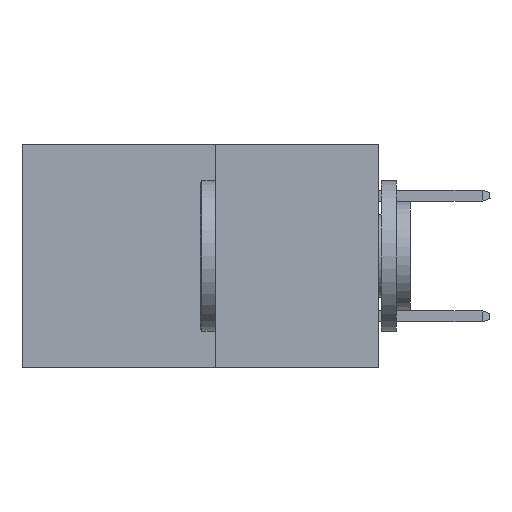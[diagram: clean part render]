
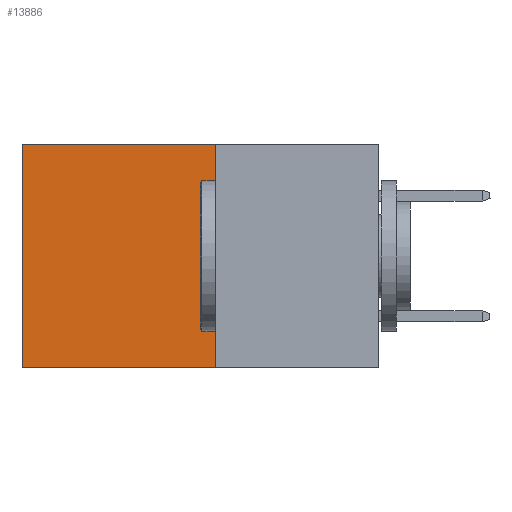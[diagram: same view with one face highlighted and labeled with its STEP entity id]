
A CAD part, left-side view. The second image highlights one B-rep face of the part: STEP entity #13886.
In plain terms, the highlighted planar face has unit normal (-1, 0, 0).
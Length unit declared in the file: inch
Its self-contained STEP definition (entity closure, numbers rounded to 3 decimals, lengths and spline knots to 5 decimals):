
#394 = AXIS2_PLACEMENT_3D ( 'NONE', #7461, #22733, #7569 ) ;
#2318 = CARTESIAN_POINT ( 'NONE',  ( 0.277, 0.59, -0.37 ) ) ;
#2329 = LINE ( 'NONE', #16534, #15059 ) ;
#3962 = ORIENTED_EDGE ( 'NONE', *, *, #25632, .T. ) ;
#4520 = ORIENTED_EDGE ( 'NONE', *, *, #11600, .T. ) ;
#5054 = PLANE ( 'NONE',  #394 ) ;
#7461 = CARTESIAN_POINT ( 'NONE',  ( 0.277, 0.27, -0.37 ) ) ;
#7485 = EDGE_CURVE ( 'NONE', #15143, #20458, #16448, .T. ) ;
#7569 = DIRECTION ( 'NONE',  ( 0., 0., -1. ) ) ;
#7715 = CARTESIAN_POINT ( 'NONE',  ( 0.277, 0.27, -0.37 ) ) ;
#9177 = DIRECTION ( 'NONE',  ( 0., 1., 0. ) ) ;
#9205 = LINE ( 'NONE', #21121, #28541 ) ;
#11600 = EDGE_CURVE ( 'NONE', #23104, #20458, #2329, .T. ) ;
#11608 = DIRECTION ( 'NONE',  ( 0., 0., -1. ) ) ;
#12657 = LINE ( 'NONE', #24418, #13428 ) ;
#12912 = VERTEX_POINT ( 'NONE', #16343 ) ;
#12972 = EDGE_LOOP ( 'NONE', ( #4520, #27186, #19836, #3962 ) ) ;
#13075 = DIRECTION ( 'NONE',  ( 0., 1., 0. ) ) ;
#13182 = CARTESIAN_POINT ( 'NONE',  ( 0.277, 0.27, -0.37 ) ) ;
#13428 = VECTOR ( 'NONE', #9177, 39.37008 ) ;
#13886 = ADVANCED_FACE ( 'NONE', ( #32751 ), #5054, .F. ) ;
#15059 = VECTOR ( 'NONE', #11608, 39.37008 ) ;
#15143 = VERTEX_POINT ( 'NONE', #7715 ) ;
#16343 = CARTESIAN_POINT ( 'NONE',  ( 0.277, 0.27, 0. ) ) ;
#16398 = CARTESIAN_POINT ( 'NONE',  ( 0.277, 0.59, 0. ) ) ;
#16448 = LINE ( 'NONE', #13182, #29089 ) ;
#16534 = CARTESIAN_POINT ( 'NONE',  ( 0.277, 0.59, -0.37 ) ) ;
#19836 = ORIENTED_EDGE ( 'NONE', *, *, #21581, .F. ) ;
#20458 = VERTEX_POINT ( 'NONE', #2318 ) ;
#21121 = CARTESIAN_POINT ( 'NONE',  ( 0.277, 0.27, -0.37 ) ) ;
#21581 = EDGE_CURVE ( 'NONE', #12912, #15143, #9205, .T. ) ;
#22733 = DIRECTION ( 'NONE',  ( 1., 0., 0. ) ) ;
#23104 = VERTEX_POINT ( 'NONE', #16398 ) ;
#23676 = DIRECTION ( 'NONE',  ( 0., 0., -1. ) ) ;
#24418 = CARTESIAN_POINT ( 'NONE',  ( 0.277, 0.27, 0. ) ) ;
#25632 = EDGE_CURVE ( 'NONE', #12912, #23104, #12657, .T. ) ;
#27186 = ORIENTED_EDGE ( 'NONE', *, *, #7485, .F. ) ;
#28541 = VECTOR ( 'NONE', #23676, 39.37008 ) ;
#29089 = VECTOR ( 'NONE', #13075, 39.37008 ) ;
#32751 = FACE_OUTER_BOUND ( 'NONE', #12972, .T. ) ;
